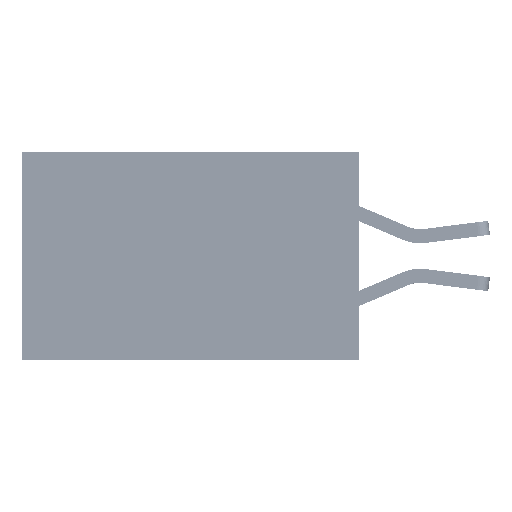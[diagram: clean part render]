
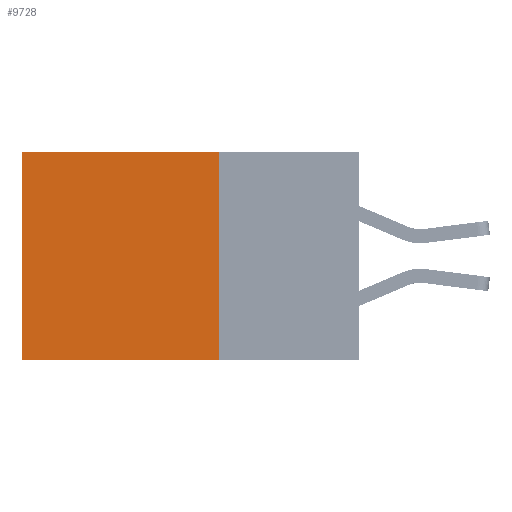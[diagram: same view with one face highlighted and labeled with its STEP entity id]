
A CAD part, left-side view. The second image highlights one B-rep face of the part: STEP entity #9728.
In plain terms, the highlighted planar face has unit normal (-1, 0, 0).
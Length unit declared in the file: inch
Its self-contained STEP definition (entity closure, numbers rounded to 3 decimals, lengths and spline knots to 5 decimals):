
#1478 = VERTEX_POINT ( 'NONE', #24692 ) ;
#2642 = CARTESIAN_POINT ( 'NONE',  ( 0.2875, 0.25, 0. ) ) ;
#2690 = AXIS2_PLACEMENT_3D ( 'NONE', #2642, #21613, #44600 ) ;
#4327 = CARTESIAN_POINT ( 'NONE',  ( 0.2875, 0.6, 0. ) ) ;
#8572 = CARTESIAN_POINT ( 'NONE',  ( 0.2875, 0.6, -0.37 ) ) ;
#9012 = CARTESIAN_POINT ( 'NONE',  ( 0.2875, 0.25, 0. ) ) ;
#9126 = VERTEX_POINT ( 'NONE', #29751 ) ;
#9728 = ADVANCED_FACE ( 'NONE', ( #10683 ), #14496, .F. ) ;
#9976 = ORIENTED_EDGE ( 'NONE', *, *, #23372, .T. ) ;
#10683 = FACE_OUTER_BOUND ( 'NONE', #35278, .T. ) ;
#14496 = PLANE ( 'NONE',  #2690 ) ;
#15562 = DIRECTION ( 'NONE',  ( 0., 1., 0. ) ) ;
#15734 = ORIENTED_EDGE ( 'NONE', *, *, #27431, .F. ) ;
#18399 = CARTESIAN_POINT ( 'NONE',  ( 0.2875, 0.25, -0.37 ) ) ;
#20894 = LINE ( 'NONE', #38532, #27382 ) ;
#21097 = VECTOR ( 'NONE', #46260, 39.37008 ) ;
#21613 = DIRECTION ( 'NONE',  ( 1., 0., 0. ) ) ;
#22212 = DIRECTION ( 'NONE',  ( 0., 1., 0. ) ) ;
#22337 = VECTOR ( 'NONE', #22212, 39.37008 ) ;
#23372 = EDGE_CURVE ( 'NONE', #9126, #44409, #20894, .T. ) ;
#24692 = CARTESIAN_POINT ( 'NONE',  ( 0.2875, 0.25, -0.37 ) ) ;
#25727 = ORIENTED_EDGE ( 'NONE', *, *, #33130, .T. ) ;
#27382 = VECTOR ( 'NONE', #15562, 39.37008 ) ;
#27431 = EDGE_CURVE ( 'NONE', #1478, #29914, #32397, .T. ) ;
#29231 = LINE ( 'NONE', #9012, #35108 ) ;
#29751 = CARTESIAN_POINT ( 'NONE',  ( 0.2875, 0.25, 0. ) ) ;
#29914 = VERTEX_POINT ( 'NONE', #8572 ) ;
#32397 = LINE ( 'NONE', #18399, #22337 ) ;
#33130 = EDGE_CURVE ( 'NONE', #44409, #29914, #37627, .T. ) ;
#33872 = ORIENTED_EDGE ( 'NONE', *, *, #47294, .F. ) ;
#35108 = VECTOR ( 'NONE', #35771, 39.37008 ) ;
#35278 = EDGE_LOOP ( 'NONE', ( #25727, #15734, #33872, #9976 ) ) ;
#35771 = DIRECTION ( 'NONE',  ( 0., 0., -1. ) ) ;
#37627 = LINE ( 'NONE', #48262, #21097 ) ;
#38532 = CARTESIAN_POINT ( 'NONE',  ( 0.2875, 0.25, 0. ) ) ;
#44409 = VERTEX_POINT ( 'NONE', #4327 ) ;
#44600 = DIRECTION ( 'NONE',  ( 0., 0., -1. ) ) ;
#46260 = DIRECTION ( 'NONE',  ( 0., 0., -1. ) ) ;
#47294 = EDGE_CURVE ( 'NONE', #9126, #1478, #29231, .T. ) ;
#48262 = CARTESIAN_POINT ( 'NONE',  ( 0.2875, 0.6, 0. ) ) ;
